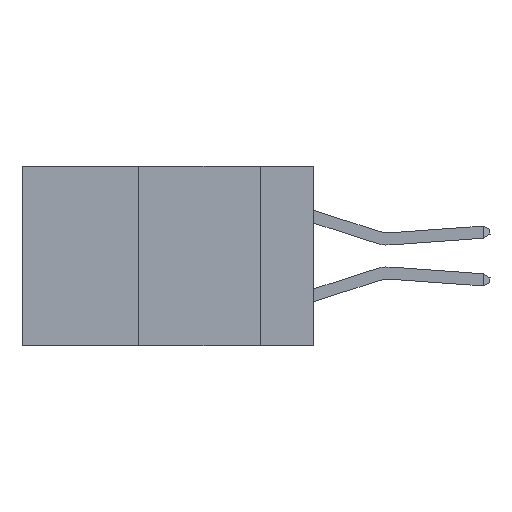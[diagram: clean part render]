
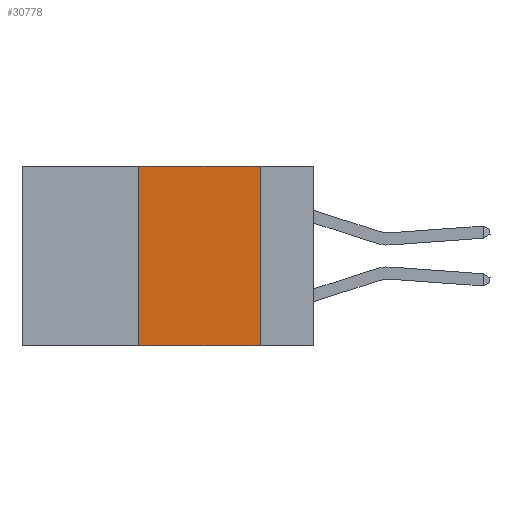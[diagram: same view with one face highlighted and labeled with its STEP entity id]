
A CAD part, left-side view. The second image highlights one B-rep face of the part: STEP entity #30778.
In plain terms, the highlighted planar face has unit normal (-1, 0, 0).
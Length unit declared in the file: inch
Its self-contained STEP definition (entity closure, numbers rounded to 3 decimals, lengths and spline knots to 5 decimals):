
#285 = LINE ( 'NONE', #5933, #33058 ) ;
#752 = DIRECTION ( 'NONE',  ( 1., 0., 0. ) ) ;
#834 = CARTESIAN_POINT ( 'NONE',  ( 0., 0.36, 0. ) ) ;
#4143 = VERTEX_POINT ( 'NONE', #9623 ) ;
#5933 = CARTESIAN_POINT ( 'NONE',  ( 0., 0.36, 0. ) ) ;
#6819 = EDGE_CURVE ( 'NONE', #28050, #4143, #20698, .T. ) ;
#7730 = CARTESIAN_POINT ( 'NONE',  ( 0., 0.36, -0.37 ) ) ;
#8767 = DIRECTION ( 'NONE',  ( 0., 0., 1. ) ) ;
#9623 = CARTESIAN_POINT ( 'NONE',  ( 0., 0.11, -0.37 ) ) ;
#11176 = VERTEX_POINT ( 'NONE', #834 ) ;
#12625 = LINE ( 'NONE', #16982, #25295 ) ;
#13390 = VECTOR ( 'NONE', #20795, 39.37008 ) ;
#14562 = DIRECTION ( 'NONE',  ( 0., -1., 0. ) ) ;
#14925 = ORIENTED_EDGE ( 'NONE', *, *, #6819, .F. ) ;
#15324 = CARTESIAN_POINT ( 'NONE',  ( 0., 0.11, 0. ) ) ;
#15512 = AXIS2_PLACEMENT_3D ( 'NONE', #33307, #752, #20274 ) ;
#16982 = CARTESIAN_POINT ( 'NONE',  ( 0., 0.6, -0.37 ) ) ;
#17680 = VECTOR ( 'NONE', #14562, 39.37008 ) ;
#19778 = VERTEX_POINT ( 'NONE', #7730 ) ;
#20128 = ORIENTED_EDGE ( 'NONE', *, *, #22306, .F. ) ;
#20274 = DIRECTION ( 'NONE',  ( 0., 0., -1. ) ) ;
#20698 = LINE ( 'NONE', #15324, #13390 ) ;
#20795 = DIRECTION ( 'NONE',  ( 0., 0., -1. ) ) ;
#22306 = EDGE_CURVE ( 'NONE', #19778, #11176, #285, .T. ) ;
#23751 = EDGE_LOOP ( 'NONE', ( #14925, #30740, #20128, #29238 ) ) ;
#24747 = LINE ( 'NONE', #25259, #17680 ) ;
#25259 = CARTESIAN_POINT ( 'NONE',  ( 0., 0.6, 0. ) ) ;
#25295 = VECTOR ( 'NONE', #30254, 39.37008 ) ;
#25672 = FACE_OUTER_BOUND ( 'NONE', #23751, .T. ) ;
#28050 = VERTEX_POINT ( 'NONE', #34700 ) ;
#29238 = ORIENTED_EDGE ( 'NONE', *, *, #30135, .T. ) ;
#30135 = EDGE_CURVE ( 'NONE', #19778, #4143, #12625, .T. ) ;
#30254 = DIRECTION ( 'NONE',  ( 0., -1., 0. ) ) ;
#30682 = PLANE ( 'NONE',  #15512 ) ;
#30740 = ORIENTED_EDGE ( 'NONE', *, *, #32040, .F. ) ;
#30778 = ADVANCED_FACE ( 'NONE', ( #25672 ), #30682, .F. ) ;
#32040 = EDGE_CURVE ( 'NONE', #11176, #28050, #24747, .T. ) ;
#33058 = VECTOR ( 'NONE', #8767, 39.37008 ) ;
#33307 = CARTESIAN_POINT ( 'NONE',  ( 0., 0.6, 0. ) ) ;
#34700 = CARTESIAN_POINT ( 'NONE',  ( 0., 0.11, 0. ) ) ;
